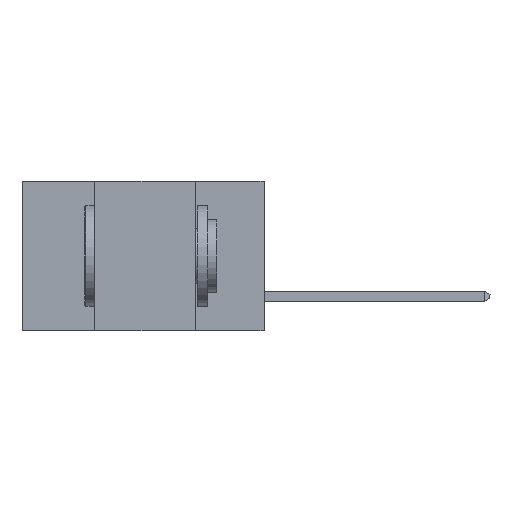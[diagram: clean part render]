
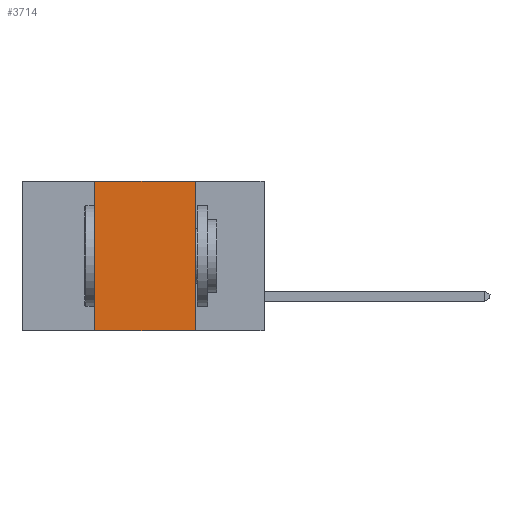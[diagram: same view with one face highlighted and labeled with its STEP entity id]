
A CAD part, left-side view. The second image highlights one B-rep face of the part: STEP entity #3714.
In plain terms, the highlighted planar face has unit normal (-1, 0, 0).
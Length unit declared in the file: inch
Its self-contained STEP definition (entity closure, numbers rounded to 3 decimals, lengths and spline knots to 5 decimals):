
#31 = CARTESIAN_POINT ( 'NONE',  ( 0., 0.17, 0. ) ) ;
#87 = LINE ( 'NONE', #802, #4823 ) ;
#457 = VERTEX_POINT ( 'NONE', #951 ) ;
#802 = CARTESIAN_POINT ( 'NONE',  ( 0., 0.6, 0. ) ) ;
#924 = DIRECTION ( 'NONE',  ( 1., 0., 0. ) ) ;
#951 = CARTESIAN_POINT ( 'NONE',  ( 0., 0.42, 0. ) ) ;
#962 = ORIENTED_EDGE ( 'NONE', *, *, #9084, .T. ) ;
#1490 = VECTOR ( 'NONE', #4362, 39.37008 ) ;
#1551 = VERTEX_POINT ( 'NONE', #9131 ) ;
#1621 = CARTESIAN_POINT ( 'NONE',  ( 0., 0.6, 0. ) ) ;
#2221 = LINE ( 'NONE', #5046, #1490 ) ;
#2260 = EDGE_CURVE ( 'NONE', #457, #8952, #87, .T. ) ;
#2317 = VECTOR ( 'NONE', #8719, 39.37008 ) ;
#2651 = AXIS2_PLACEMENT_3D ( 'NONE', #1621, #924, #7850 ) ;
#2952 = CARTESIAN_POINT ( 'NONE',  ( 0., 0.6, -0.37 ) ) ;
#3051 = EDGE_LOOP ( 'NONE', ( #6123, #8096, #6181, #962 ) ) ;
#3240 = VECTOR ( 'NONE', #6641, 39.37008 ) ;
#3343 = EDGE_CURVE ( 'NONE', #8952, #8964, #7508, .T. ) ;
#3637 = DIRECTION ( 'NONE',  ( 0., -1., 0. ) ) ;
#3709 = PLANE ( 'NONE',  #2651 ) ;
#3714 = ADVANCED_FACE ( 'NONE', ( #8631 ), #3709, .F. ) ;
#4355 = LINE ( 'NONE', #2952, #2317 ) ;
#4362 = DIRECTION ( 'NONE',  ( 0., 0., 1. ) ) ;
#4823 = VECTOR ( 'NONE', #3637, 39.37008 ) ;
#5019 = EDGE_CURVE ( 'NONE', #1551, #457, #2221, .T. ) ;
#5046 = CARTESIAN_POINT ( 'NONE',  ( 0., 0.42, -0.37 ) ) ;
#5990 = CARTESIAN_POINT ( 'NONE',  ( 0., 0.17, -0.37 ) ) ;
#6123 = ORIENTED_EDGE ( 'NONE', *, *, #3343, .F. ) ;
#6181 = ORIENTED_EDGE ( 'NONE', *, *, #5019, .F. ) ;
#6641 = DIRECTION ( 'NONE',  ( 0., 0., -1. ) ) ;
#7508 = LINE ( 'NONE', #5990, #3240 ) ;
#7850 = DIRECTION ( 'NONE',  ( 0., 0., -1. ) ) ;
#8096 = ORIENTED_EDGE ( 'NONE', *, *, #2260, .F. ) ;
#8365 = CARTESIAN_POINT ( 'NONE',  ( 0., 0.17, -0.37 ) ) ;
#8631 = FACE_OUTER_BOUND ( 'NONE', #3051, .T. ) ;
#8719 = DIRECTION ( 'NONE',  ( 0., -1., 0. ) ) ;
#8952 = VERTEX_POINT ( 'NONE', #31 ) ;
#8964 = VERTEX_POINT ( 'NONE', #8365 ) ;
#9084 = EDGE_CURVE ( 'NONE', #1551, #8964, #4355, .T. ) ;
#9131 = CARTESIAN_POINT ( 'NONE',  ( 0., 0.42, -0.37 ) ) ;
